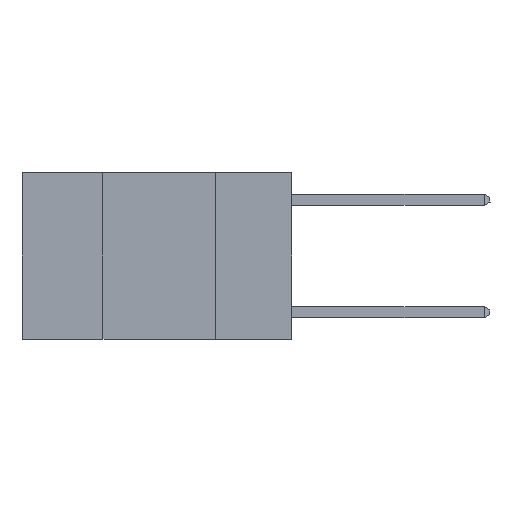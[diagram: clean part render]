
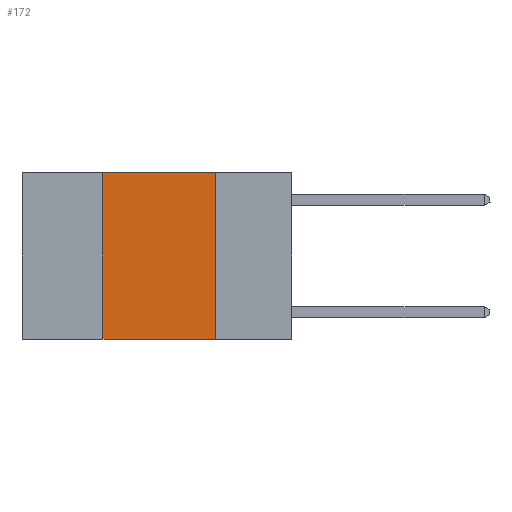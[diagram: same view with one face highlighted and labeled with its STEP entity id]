
A CAD part, left-side view. The second image highlights one B-rep face of the part: STEP entity #172.
In plain terms, the highlighted planar face has unit normal (-1, 0, 0).
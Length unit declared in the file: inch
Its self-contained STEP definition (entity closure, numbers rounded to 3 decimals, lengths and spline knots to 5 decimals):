
#172 = ADVANCED_FACE ( 'NONE', ( #25414 ), #1933, .F. ) ;
#1933 = PLANE ( 'NONE',  #4348 ) ;
#2822 = CARTESIAN_POINT ( 'NONE',  ( 0., 0.17, 0. ) ) ;
#3573 = VERTEX_POINT ( 'NONE', #8628 ) ;
#4022 = EDGE_CURVE ( 'NONE', #13725, #3573, #27654, .T. ) ;
#4280 = DIRECTION ( 'NONE',  ( 1., 0., 0. ) ) ;
#4285 = VECTOR ( 'NONE', #18336, 39.37008 ) ;
#4348 = AXIS2_PLACEMENT_3D ( 'NONE', #22335, #4280, #20230 ) ;
#5439 = CARTESIAN_POINT ( 'NONE',  ( 0., 0.6, -0.37 ) ) ;
#5765 = EDGE_CURVE ( 'NONE', #5941, #28018, #23073, .T. ) ;
#5863 = ORIENTED_EDGE ( 'NONE', *, *, #5765, .F. ) ;
#5941 = VERTEX_POINT ( 'NONE', #7520 ) ;
#7520 = CARTESIAN_POINT ( 'NONE',  ( 0., 0.42, 0. ) ) ;
#8628 = CARTESIAN_POINT ( 'NONE',  ( 0., 0.17, -0.37 ) ) ;
#9035 = VECTOR ( 'NONE', #12269, 39.37008 ) ;
#9292 = DIRECTION ( 'NONE',  ( 0., 0., 1. ) ) ;
#12269 = DIRECTION ( 'NONE',  ( 0., -1., 0. ) ) ;
#12704 = ORIENTED_EDGE ( 'NONE', *, *, #28722, .F. ) ;
#13725 = VERTEX_POINT ( 'NONE', #20241 ) ;
#15058 = LINE ( 'NONE', #2822, #26193 ) ;
#16038 = CARTESIAN_POINT ( 'NONE',  ( 0., 0.6, 0. ) ) ;
#16742 = VECTOR ( 'NONE', #9292, 39.37008 ) ;
#18174 = DIRECTION ( 'NONE',  ( 0., 0., -1. ) ) ;
#18336 = DIRECTION ( 'NONE',  ( 0., -1., 0. ) ) ;
#18723 = ORIENTED_EDGE ( 'NONE', *, *, #4022, .T. ) ;
#19282 = EDGE_LOOP ( 'NONE', ( #23179, #5863, #12704, #18723 ) ) ;
#20230 = DIRECTION ( 'NONE',  ( 0., 0., -1. ) ) ;
#20241 = CARTESIAN_POINT ( 'NONE',  ( 0., 0.42, -0.37 ) ) ;
#20605 = CARTESIAN_POINT ( 'NONE',  ( 0., 0.42, 0. ) ) ;
#22335 = CARTESIAN_POINT ( 'NONE',  ( 0., 0.6, 0. ) ) ;
#22628 = LINE ( 'NONE', #20605, #16742 ) ;
#22833 = CARTESIAN_POINT ( 'NONE',  ( 0., 0.17, 0. ) ) ;
#23073 = LINE ( 'NONE', #16038, #4285 ) ;
#23179 = ORIENTED_EDGE ( 'NONE', *, *, #27285, .F. ) ;
#25414 = FACE_OUTER_BOUND ( 'NONE', #19282, .T. ) ;
#26193 = VECTOR ( 'NONE', #18174, 39.37008 ) ;
#27285 = EDGE_CURVE ( 'NONE', #28018, #3573, #15058, .T. ) ;
#27654 = LINE ( 'NONE', #5439, #9035 ) ;
#28018 = VERTEX_POINT ( 'NONE', #22833 ) ;
#28722 = EDGE_CURVE ( 'NONE', #13725, #5941, #22628, .T. ) ;
